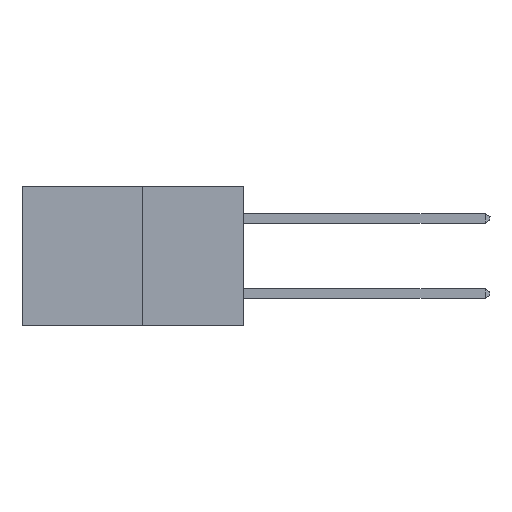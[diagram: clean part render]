
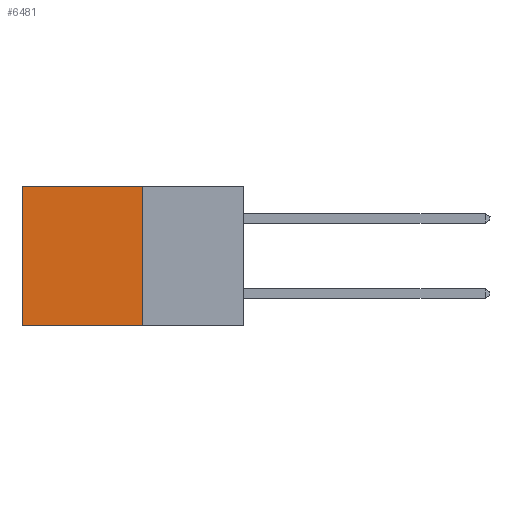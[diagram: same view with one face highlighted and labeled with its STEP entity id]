
A CAD part, left-side view. The second image highlights one B-rep face of the part: STEP entity #6481.
In plain terms, the highlighted planar face has unit normal (-1, 0, 0).
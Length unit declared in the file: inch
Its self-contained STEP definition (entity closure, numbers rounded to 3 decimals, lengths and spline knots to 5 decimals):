
#77 = EDGE_CURVE ( 'NONE', #14146, #1313, #12888, .T. ) ;
#144 = EDGE_CURVE ( 'NONE', #14146, #4744, #5028, .T. ) ;
#159 = DIRECTION ( 'NONE',  ( 1., 0., 0. ) ) ;
#1000 = VECTOR ( 'NONE', #11155, 39.37008 ) ;
#1188 = CARTESIAN_POINT ( 'NONE',  ( 0.277, 0.59, 0. ) ) ;
#1313 = VERTEX_POINT ( 'NONE', #1188 ) ;
#2241 = ORIENTED_EDGE ( 'NONE', *, *, #9897, .T. ) ;
#2433 = EDGE_CURVE ( 'NONE', #4744, #5493, #16328, .T. ) ;
#2844 = CARTESIAN_POINT ( 'NONE',  ( 0.277, 0.59, -0.37 ) ) ;
#3026 = VECTOR ( 'NONE', #4225, 39.37008 ) ;
#4225 = DIRECTION ( 'NONE',  ( 0., 0., -1. ) ) ;
#4369 = ORIENTED_EDGE ( 'NONE', *, *, #144, .F. ) ;
#4744 = VERTEX_POINT ( 'NONE', #18192 ) ;
#5028 = LINE ( 'NONE', #7489, #7554 ) ;
#5277 = EDGE_LOOP ( 'NONE', ( #2241, #9295, #4369, #9961 ) ) ;
#5385 = VECTOR ( 'NONE', #9838, 39.37008 ) ;
#5493 = VERTEX_POINT ( 'NONE', #2844 ) ;
#6481 = ADVANCED_FACE ( 'NONE', ( #12675 ), #16599, .F. ) ;
#7489 = CARTESIAN_POINT ( 'NONE',  ( 0.277, 0.27, -0.37 ) ) ;
#7554 = VECTOR ( 'NONE', #13672, 39.37008 ) ;
#9158 = CARTESIAN_POINT ( 'NONE',  ( 0.277, 0.27, -0.37 ) ) ;
#9295 = ORIENTED_EDGE ( 'NONE', *, *, #2433, .F. ) ;
#9838 = DIRECTION ( 'NONE',  ( 0., 1., 0. ) ) ;
#9897 = EDGE_CURVE ( 'NONE', #1313, #5493, #13943, .T. ) ;
#9961 = ORIENTED_EDGE ( 'NONE', *, *, #77, .T. ) ;
#10304 = CARTESIAN_POINT ( 'NONE',  ( 0.277, 0.27, -0.37 ) ) ;
#10650 = DIRECTION ( 'NONE',  ( 0., 0., -1. ) ) ;
#11155 = DIRECTION ( 'NONE',  ( 0., 1., 0. ) ) ;
#12633 = AXIS2_PLACEMENT_3D ( 'NONE', #9158, #159, #10650 ) ;
#12675 = FACE_OUTER_BOUND ( 'NONE', #5277, .T. ) ;
#12888 = LINE ( 'NONE', #16740, #1000 ) ;
#13084 = CARTESIAN_POINT ( 'NONE',  ( 0.277, 0.59, -0.37 ) ) ;
#13672 = DIRECTION ( 'NONE',  ( 0., 0., -1. ) ) ;
#13736 = CARTESIAN_POINT ( 'NONE',  ( 0.277, 0.27, 0. ) ) ;
#13943 = LINE ( 'NONE', #13084, #3026 ) ;
#14146 = VERTEX_POINT ( 'NONE', #13736 ) ;
#16328 = LINE ( 'NONE', #10304, #5385 ) ;
#16599 = PLANE ( 'NONE',  #12633 ) ;
#16740 = CARTESIAN_POINT ( 'NONE',  ( 0.277, 0.27, 0. ) ) ;
#18192 = CARTESIAN_POINT ( 'NONE',  ( 0.277, 0.27, -0.37 ) ) ;
